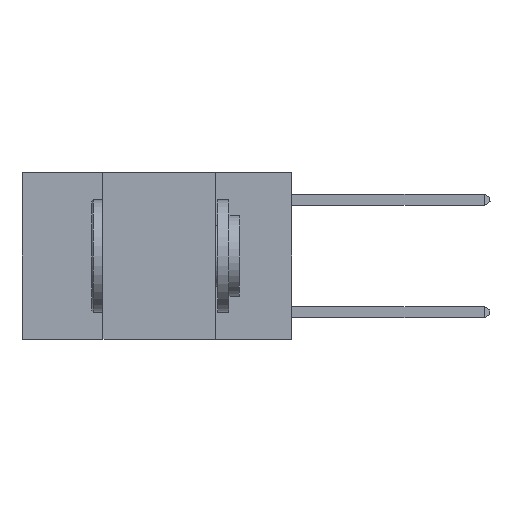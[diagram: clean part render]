
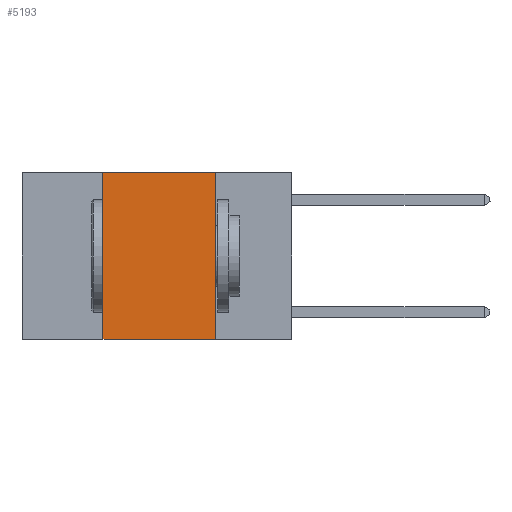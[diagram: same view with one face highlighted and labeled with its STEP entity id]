
A CAD part, left-side view. The second image highlights one B-rep face of the part: STEP entity #5193.
In plain terms, the highlighted planar face has unit normal (-1, 0, 0).
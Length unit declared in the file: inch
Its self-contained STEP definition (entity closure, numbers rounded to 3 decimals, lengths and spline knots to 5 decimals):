
#259 = ORIENTED_EDGE ( 'NONE', *, *, #8194, .F. ) ;
#272 = ORIENTED_EDGE ( 'NONE', *, *, #6923, .F. ) ;
#284 = ORIENTED_EDGE ( 'NONE', *, *, #6523, .T. ) ;
#413 = DIRECTION ( 'NONE',  ( 0., -1., 0. ) ) ;
#1263 = AXIS2_PLACEMENT_3D ( 'NONE', #4057, #9189, #4857 ) ;
#1329 = ORIENTED_EDGE ( 'NONE', *, *, #5456, .F. ) ;
#1676 = LINE ( 'NONE', #4373, #5682 ) ;
#1803 = FACE_OUTER_BOUND ( 'NONE', #3551, .T. ) ;
#1811 = CARTESIAN_POINT ( 'NONE',  ( 0., 0.42, -0.37 ) ) ;
#2370 = CARTESIAN_POINT ( 'NONE',  ( 0., 0.6, -0.37 ) ) ;
#2568 = VERTEX_POINT ( 'NONE', #6941 ) ;
#2759 = DIRECTION ( 'NONE',  ( 0., 0., -1. ) ) ;
#3245 = VERTEX_POINT ( 'NONE', #1811 ) ;
#3551 = EDGE_LOOP ( 'NONE', ( #1329, #259, #272, #284 ) ) ;
#4033 = VECTOR ( 'NONE', #9427, 39.37008 ) ;
#4057 = CARTESIAN_POINT ( 'NONE',  ( 0., 0.6, 0. ) ) ;
#4373 = CARTESIAN_POINT ( 'NONE',  ( 0., 0.17, 0. ) ) ;
#4857 = DIRECTION ( 'NONE',  ( 0., 0., -1. ) ) ;
#5022 = CARTESIAN_POINT ( 'NONE',  ( 0., 0.17, 0. ) ) ;
#5193 = ADVANCED_FACE ( 'NONE', ( #1803 ), #6316, .F. ) ;
#5456 = EDGE_CURVE ( 'NONE', #8054, #2568, #1676, .T. ) ;
#5512 = DIRECTION ( 'NONE',  ( 0., -1., 0. ) ) ;
#5682 = VECTOR ( 'NONE', #2759, 39.37008 ) ;
#5953 = VECTOR ( 'NONE', #5512, 39.37008 ) ;
#6189 = VERTEX_POINT ( 'NONE', #6718 ) ;
#6316 = PLANE ( 'NONE',  #1263 ) ;
#6523 = EDGE_CURVE ( 'NONE', #3245, #2568, #9737, .T. ) ;
#6718 = CARTESIAN_POINT ( 'NONE',  ( 0., 0.42, 0. ) ) ;
#6923 = EDGE_CURVE ( 'NONE', #3245, #6189, #9405, .T. ) ;
#6941 = CARTESIAN_POINT ( 'NONE',  ( 0., 0.17, -0.37 ) ) ;
#8039 = LINE ( 'NONE', #9568, #9695 ) ;
#8054 = VERTEX_POINT ( 'NONE', #5022 ) ;
#8194 = EDGE_CURVE ( 'NONE', #6189, #8054, #8039, .T. ) ;
#8716 = CARTESIAN_POINT ( 'NONE',  ( 0., 0.42, 0. ) ) ;
#9189 = DIRECTION ( 'NONE',  ( 1., 0., 0. ) ) ;
#9405 = LINE ( 'NONE', #8716, #4033 ) ;
#9427 = DIRECTION ( 'NONE',  ( 0., 0., 1. ) ) ;
#9568 = CARTESIAN_POINT ( 'NONE',  ( 0., 0.6, 0. ) ) ;
#9695 = VECTOR ( 'NONE', #413, 39.37008 ) ;
#9737 = LINE ( 'NONE', #2370, #5953 ) ;
